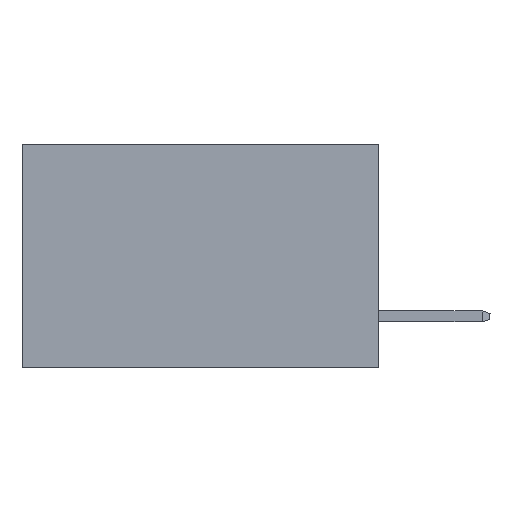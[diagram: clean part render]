
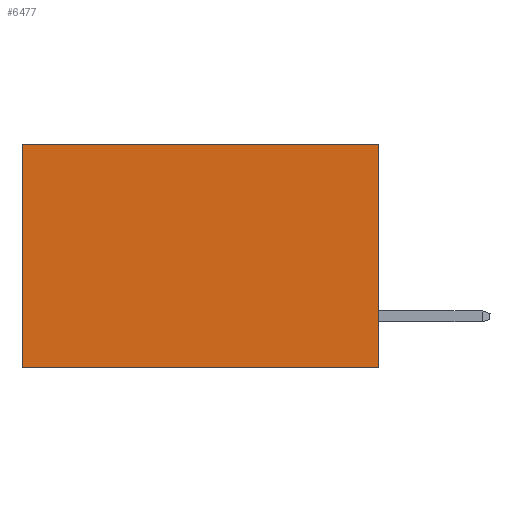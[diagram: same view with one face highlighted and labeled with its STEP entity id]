
A CAD part, left-side view. The second image highlights one B-rep face of the part: STEP entity #6477.
In plain terms, the highlighted planar face has unit normal (-1, 0, 0).
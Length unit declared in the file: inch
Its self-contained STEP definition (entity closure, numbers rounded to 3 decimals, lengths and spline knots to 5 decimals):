
#90 = CARTESIAN_POINT ( 'NONE',  ( 0.277, 0., -0.37 ) ) ;
#237 = FACE_OUTER_BOUND ( 'NONE', #526, .T. ) ;
#362 = EDGE_CURVE ( 'NONE', #8970, #1429, #10400, .T. ) ;
#416 = CARTESIAN_POINT ( 'NONE',  ( 0.277, 0.59, -0.37 ) ) ;
#526 = EDGE_LOOP ( 'NONE', ( #7146, #7163, #7171, #7263 ) ) ;
#856 = EDGE_CURVE ( 'NONE', #1429, #2304, #9807, .T. ) ;
#1429 = VERTEX_POINT ( 'NONE', #2387 ) ;
#1444 = CARTESIAN_POINT ( 'NONE',  ( 0.277, 0., -0.37 ) ) ;
#2024 = EDGE_CURVE ( 'NONE', #4126, #2304, #3489, .T. ) ;
#2080 = EDGE_CURVE ( 'NONE', #8970, #4126, #8653, .T. ) ;
#2304 = VERTEX_POINT ( 'NONE', #6656 ) ;
#2335 = VECTOR ( 'NONE', #9102, 39.37008 ) ;
#2387 = CARTESIAN_POINT ( 'NONE',  ( 0.277, 0.59, 0. ) ) ;
#3434 = DIRECTION ( 'NONE',  ( 0., 0., -1. ) ) ;
#3452 = DIRECTION ( 'NONE',  ( 1., 0., 0. ) ) ;
#3489 = LINE ( 'NONE', #9510, #7208 ) ;
#4126 = VERTEX_POINT ( 'NONE', #1444 ) ;
#4868 = CARTESIAN_POINT ( 'NONE',  ( 0.277, 0., -0.37 ) ) ;
#4876 = PLANE ( 'NONE',  #9713 ) ;
#5474 = VECTOR ( 'NONE', #10504, 39.37008 ) ;
#6477 = ADVANCED_FACE ( 'NONE', ( #237 ), #4876, .F. ) ;
#6656 = CARTESIAN_POINT ( 'NONE',  ( 0.277, 0.59, -0.37 ) ) ;
#7146 = ORIENTED_EDGE ( 'NONE', *, *, #856, .T. ) ;
#7163 = ORIENTED_EDGE ( 'NONE', *, *, #2024, .F. ) ;
#7171 = ORIENTED_EDGE ( 'NONE', *, *, #2080, .F. ) ;
#7208 = VECTOR ( 'NONE', #9951, 39.37008 ) ;
#7263 = ORIENTED_EDGE ( 'NONE', *, *, #362, .T. ) ;
#7801 = DIRECTION ( 'NONE',  ( 0., 1., 0. ) ) ;
#8308 = VECTOR ( 'NONE', #7801, 39.37008 ) ;
#8653 = LINE ( 'NONE', #90, #2335 ) ;
#8900 = CARTESIAN_POINT ( 'NONE',  ( 0.277, 0., 0. ) ) ;
#8970 = VERTEX_POINT ( 'NONE', #8900 ) ;
#9102 = DIRECTION ( 'NONE',  ( 0., 0., -1. ) ) ;
#9510 = CARTESIAN_POINT ( 'NONE',  ( 0.277, 0., -0.37 ) ) ;
#9713 = AXIS2_PLACEMENT_3D ( 'NONE', #4868, #3452, #3434 ) ;
#9807 = LINE ( 'NONE', #416, #5474 ) ;
#9951 = DIRECTION ( 'NONE',  ( 0., 1., 0. ) ) ;
#10286 = CARTESIAN_POINT ( 'NONE',  ( 0.277, 0., 0. ) ) ;
#10400 = LINE ( 'NONE', #10286, #8308 ) ;
#10504 = DIRECTION ( 'NONE',  ( 0., 0., -1. ) ) ;
